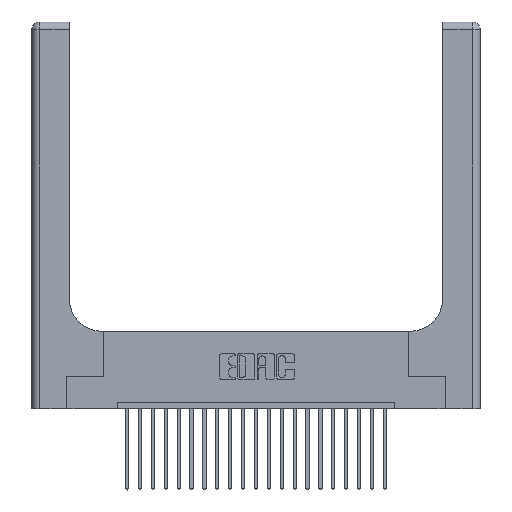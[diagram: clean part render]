
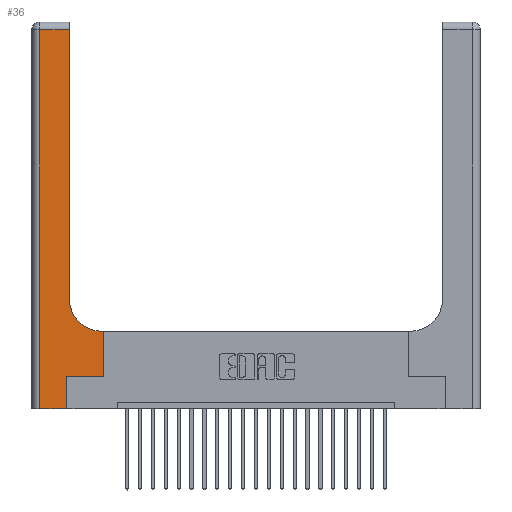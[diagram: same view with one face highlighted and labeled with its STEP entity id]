
A CAD part, top view. The second image highlights one B-rep face of the part: STEP entity #36.
In plain terms, the highlighted planar face has unit normal (0, 0, 1).
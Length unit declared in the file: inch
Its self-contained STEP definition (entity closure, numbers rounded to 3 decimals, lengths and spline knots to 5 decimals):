
#36 = ADVANCED_FACE ( 'NONE', ( #2619 ), #17770, .F. ) ;
#149 = DIRECTION ( 'NONE',  ( 0., 0., -1. ) ) ;
#336 = CARTESIAN_POINT ( 'NONE',  ( 0., 2.94, 0.37 ) ) ;
#480 = CARTESIAN_POINT ( 'NONE',  ( 0.269, 0., 0.37 ) ) ;
#557 = ORIENTED_EDGE ( 'NONE', *, *, #16048, .T. ) ;
#1008 = CARTESIAN_POINT ( 'NONE',  ( 0.269, 0.25, 0.37 ) ) ;
#1771 = CARTESIAN_POINT ( 'NONE',  ( 0.5585, 0.6, 0.37 ) ) ;
#1838 = EDGE_CURVE ( 'NONE', #13006, #10137, #19759, .T. ) ;
#2501 = CARTESIAN_POINT ( 'NONE',  ( 0.06, 0., 0.37 ) ) ;
#2619 = FACE_OUTER_BOUND ( 'NONE', #22597, .T. ) ;
#2722 = CARTESIAN_POINT ( 'NONE',  ( 0.5415, 0.85, 0.37 ) ) ;
#3041 = ORIENTED_EDGE ( 'NONE', *, *, #22964, .T. ) ;
#3161 = VERTEX_POINT ( 'NONE', #6282 ) ;
#3819 = CARTESIAN_POINT ( 'NONE',  ( 0.5585, 0.25, 0.37 ) ) ;
#4166 = DIRECTION ( 'NONE',  ( 0., 1., 0. ) ) ;
#5170 = LINE ( 'NONE', #6811, #17260 ) ;
#5370 = EDGE_CURVE ( 'NONE', #17657, #3161, #12996, .T. ) ;
#5755 = LINE ( 'NONE', #22319, #20764 ) ;
#5959 = DIRECTION ( 'NONE',  ( 1., 0., 0. ) ) ;
#6007 = EDGE_CURVE ( 'NONE', #8774, #17657, #5755, .T. ) ;
#6282 = CARTESIAN_POINT ( 'NONE',  ( 0.269, 0., 0.37 ) ) ;
#6376 = VERTEX_POINT ( 'NONE', #9634 ) ;
#6414 = EDGE_CURVE ( 'NONE', #17337, #13006, #5170, .T. ) ;
#6440 = LINE ( 'NONE', #480, #19376 ) ;
#6811 = CARTESIAN_POINT ( 'NONE',  ( 0.2915, 0.6, 0.37 ) ) ;
#6823 = ORIENTED_EDGE ( 'NONE', *, *, #1838, .T. ) ;
#6880 = VERTEX_POINT ( 'NONE', #19958 ) ;
#6963 = LINE ( 'NONE', #22759, #7523 ) ;
#7075 = CARTESIAN_POINT ( 'NONE',  ( 0.5415, 0.6, 0.37 ) ) ;
#7523 = VECTOR ( 'NONE', #4166, 39.37008 ) ;
#8108 = VECTOR ( 'NONE', #19875, 39.37008 ) ;
#8774 = VERTEX_POINT ( 'NONE', #11653 ) ;
#9259 = DIRECTION ( 'NONE',  ( 0., -1., 0. ) ) ;
#9309 = ORIENTED_EDGE ( 'NONE', *, *, #19204, .T. ) ;
#9458 = DIRECTION ( 'NONE',  ( 0., 1., 0. ) ) ;
#9634 = CARTESIAN_POINT ( 'NONE',  ( 0.269, 0.25, 0.37 ) ) ;
#9953 = EDGE_CURVE ( 'NONE', #3161, #6376, #6440, .T. ) ;
#10137 = VERTEX_POINT ( 'NONE', #17808 ) ;
#11056 = ORIENTED_EDGE ( 'NONE', *, *, #6414, .T. ) ;
#11653 = CARTESIAN_POINT ( 'NONE',  ( 0.06, 2.94, 0.37 ) ) ;
#12227 = AXIS2_PLACEMENT_3D ( 'NONE', #2722, #13493, #19058 ) ;
#12321 = LINE ( 'NONE', #20227, #16882 ) ;
#12330 = CARTESIAN_POINT ( 'NONE',  ( 0., 0., 0.37 ) ) ;
#12465 = VECTOR ( 'NONE', #5959, 39.37008 ) ;
#12757 = LINE ( 'NONE', #1008, #12465 ) ;
#12996 = LINE ( 'NONE', #12330, #8108 ) ;
#13006 = VERTEX_POINT ( 'NONE', #7075 ) ;
#13493 = DIRECTION ( 'NONE',  ( 0., 0., -1. ) ) ;
#14293 = EDGE_CURVE ( 'NONE', #6880, #8774, #19296, .T. ) ;
#14487 = DIRECTION ( 'NONE',  ( 0., 1., 0. ) ) ;
#15063 = ORIENTED_EDGE ( 'NONE', *, *, #6007, .T. ) ;
#15274 = AXIS2_PLACEMENT_3D ( 'NONE', #15926, #149, #23731 ) ;
#15926 = CARTESIAN_POINT ( 'NONE',  ( 0., 3., 0.37 ) ) ;
#16048 = EDGE_CURVE ( 'NONE', #10137, #6880, #12321, .T. ) ;
#16164 = ORIENTED_EDGE ( 'NONE', *, *, #5370, .T. ) ;
#16655 = VECTOR ( 'NONE', #18751, 39.37008 ) ;
#16882 = VECTOR ( 'NONE', #14487, 39.37008 ) ;
#17260 = VECTOR ( 'NONE', #23159, 39.37008 ) ;
#17337 = VERTEX_POINT ( 'NONE', #1771 ) ;
#17657 = VERTEX_POINT ( 'NONE', #2501 ) ;
#17770 = PLANE ( 'NONE',  #15274 ) ;
#17808 = CARTESIAN_POINT ( 'NONE',  ( 0.2915, 0.85, 0.37 ) ) ;
#18751 = DIRECTION ( 'NONE',  ( -1., 0., 0. ) ) ;
#19058 = DIRECTION ( 'NONE',  ( 1., 0., 0. ) ) ;
#19060 = VERTEX_POINT ( 'NONE', #3819 ) ;
#19204 = EDGE_CURVE ( 'NONE', #6376, #19060, #12757, .T. ) ;
#19296 = LINE ( 'NONE', #336, #16655 ) ;
#19376 = VECTOR ( 'NONE', #9458, 39.37008 ) ;
#19593 = ORIENTED_EDGE ( 'NONE', *, *, #9953, .T. ) ;
#19759 = CIRCLE ( 'NONE', #12227, 0.25 ) ;
#19875 = DIRECTION ( 'NONE',  ( 1., 0., 0. ) ) ;
#19958 = CARTESIAN_POINT ( 'NONE',  ( 0.2915, 2.94, 0.37 ) ) ;
#20227 = CARTESIAN_POINT ( 'NONE',  ( 0.2915, 3., 0.37 ) ) ;
#20764 = VECTOR ( 'NONE', #9259, 39.37008 ) ;
#21778 = ORIENTED_EDGE ( 'NONE', *, *, #14293, .T. ) ;
#22319 = CARTESIAN_POINT ( 'NONE',  ( 0.06, 3., 0.37 ) ) ;
#22597 = EDGE_LOOP ( 'NONE', ( #557, #21778, #15063, #16164, #19593, #9309, #3041, #11056, #6823 ) ) ;
#22759 = CARTESIAN_POINT ( 'NONE',  ( 0.5585, 0.25, 0.37 ) ) ;
#22964 = EDGE_CURVE ( 'NONE', #19060, #17337, #6963, .T. ) ;
#23159 = DIRECTION ( 'NONE',  ( -1., 0., 0. ) ) ;
#23731 = DIRECTION ( 'NONE',  ( -1., 0., 0. ) ) ;
